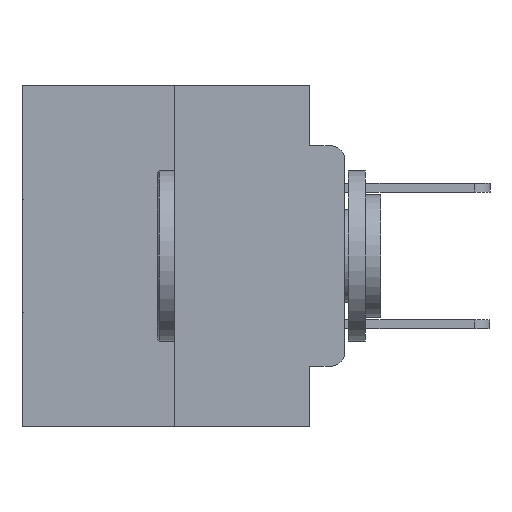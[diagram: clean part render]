
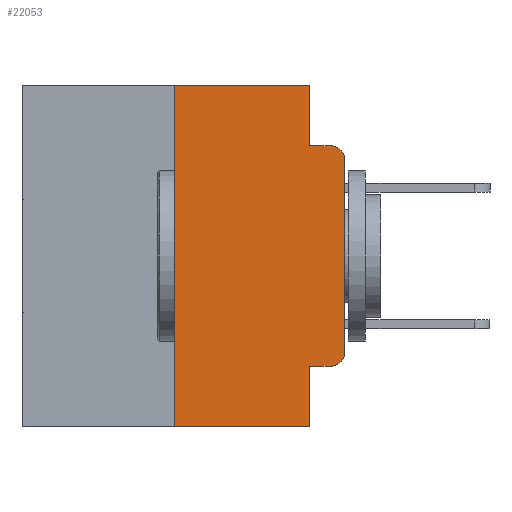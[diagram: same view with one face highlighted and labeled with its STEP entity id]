
A CAD part, left-side view. The second image highlights one B-rep face of the part: STEP entity #22053.
In plain terms, the highlighted planar face has unit normal (-1, 0, 0).
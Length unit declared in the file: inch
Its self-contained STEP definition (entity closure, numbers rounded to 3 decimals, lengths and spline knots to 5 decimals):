
#342 = EDGE_LOOP ( 'NONE', ( #15551, #16254, #22757, #11785, #12450, #8671, #27499, #22422, #17977, #758 ) ) ;
#758 = ORIENTED_EDGE ( 'NONE', *, *, #17374, .T. ) ;
#1546 = DIRECTION ( 'NONE',  ( -1., 0., 0. ) ) ;
#2364 = FACE_OUTER_BOUND ( 'NONE', #342, .T. ) ;
#2388 = EDGE_CURVE ( 'NONE', #22418, #22709, #19149, .T. ) ;
#2465 = VERTEX_POINT ( 'NONE', #24366 ) ;
#3047 = VERTEX_POINT ( 'NONE', #22172 ) ;
#3096 = EDGE_CURVE ( 'NONE', #23798, #15438, #18480, .T. ) ;
#3315 = CARTESIAN_POINT ( 'NONE',  ( 0., 0.051, 0. ) ) ;
#3863 = CARTESIAN_POINT ( 'NONE',  ( 0., 0.473, 0. ) ) ;
#3922 = EDGE_CURVE ( 'NONE', #22709, #2465, #4862, .T. ) ;
#4197 = CARTESIAN_POINT ( 'NONE',  ( 0., 0.051, -0.0885 ) ) ;
#4744 = AXIS2_PLACEMENT_3D ( 'NONE', #18377, #5075, #20560 ) ;
#4862 = CIRCLE ( 'NONE', #20282, 0.02 ) ;
#5075 = DIRECTION ( 'NONE',  ( -1., 0., 0. ) ) ;
#5249 = VECTOR ( 'NONE', #15201, 39.37008 ) ;
#6132 = VECTOR ( 'NONE', #8450, 39.37008 ) ;
#6475 = DIRECTION ( 'NONE',  ( 0., -1., 0. ) ) ;
#6972 = EDGE_CURVE ( 'NONE', #18510, #2465, #7589, .T. ) ;
#7490 = EDGE_CURVE ( 'NONE', #7613, #11094, #17935, .T. ) ;
#7589 = LINE ( 'NONE', #4197, #24434 ) ;
#7613 = VERTEX_POINT ( 'NONE', #28527 ) ;
#7895 = VECTOR ( 'NONE', #13419, 39.37008 ) ;
#8450 = DIRECTION ( 'NONE',  ( 0., -1., 0. ) ) ;
#8636 = CARTESIAN_POINT ( 'NONE',  ( 0., 0., 0. ) ) ;
#8671 = ORIENTED_EDGE ( 'NONE', *, *, #11474, .F. ) ;
#8853 = PLANE ( 'NONE',  #14910 ) ;
#8885 = VECTOR ( 'NONE', #16711, 39.37008 ) ;
#8913 = CARTESIAN_POINT ( 'NONE',  ( 0., 0., -0.1085 ) ) ;
#8957 = CARTESIAN_POINT ( 'NONE',  ( 0., 0.051, -0.5 ) ) ;
#9612 = DIRECTION ( 'NONE',  ( 0., 0., 1. ) ) ;
#10019 = EDGE_CURVE ( 'NONE', #11094, #18510, #19877, .T. ) ;
#11094 = VERTEX_POINT ( 'NONE', #26860 ) ;
#11159 = DIRECTION ( 'NONE',  ( 1., 0., 0. ) ) ;
#11474 = EDGE_CURVE ( 'NONE', #23798, #7613, #27956, .T. ) ;
#11785 = ORIENTED_EDGE ( 'NONE', *, *, #10019, .F. ) ;
#11928 = VECTOR ( 'NONE', #20236, 39.37008 ) ;
#12450 = ORIENTED_EDGE ( 'NONE', *, *, #7490, .F. ) ;
#12606 = VECTOR ( 'NONE', #9612, 39.37008 ) ;
#12943 = EDGE_CURVE ( 'NONE', #23839, #15438, #19624, .T. ) ;
#12982 = CARTESIAN_POINT ( 'NONE',  ( 0., 0.25, 0. ) ) ;
#13419 = DIRECTION ( 'NONE',  ( 0., 0., -1. ) ) ;
#14834 = CARTESIAN_POINT ( 'NONE',  ( 0., 0.051, -0.0885 ) ) ;
#14910 = AXIS2_PLACEMENT_3D ( 'NONE', #24271, #11159, #26454 ) ;
#15017 = CARTESIAN_POINT ( 'NONE',  ( 0., 0.02, -0.1085 ) ) ;
#15201 = DIRECTION ( 'NONE',  ( 0., 0., 1. ) ) ;
#15438 = VERTEX_POINT ( 'NONE', #8957 ) ;
#15551 = ORIENTED_EDGE ( 'NONE', *, *, #2388, .T. ) ;
#15555 = DIRECTION ( 'NONE',  ( 0., -1., 0. ) ) ;
#15620 = CARTESIAN_POINT ( 'NONE',  ( 0., 0.051, 0. ) ) ;
#15908 = EDGE_CURVE ( 'NONE', #23839, #3047, #22592, .T. ) ;
#16254 = ORIENTED_EDGE ( 'NONE', *, *, #3922, .T. ) ;
#16711 = DIRECTION ( 'NONE',  ( 0., 0., -1. ) ) ;
#17211 = DIRECTION ( 'NONE',  ( 0., 0., -1. ) ) ;
#17374 = EDGE_CURVE ( 'NONE', #3047, #22418, #19744, .T. ) ;
#17444 = VECTOR ( 'NONE', #15555, 39.37008 ) ;
#17935 = LINE ( 'NONE', #3863, #6132 ) ;
#17977 = ORIENTED_EDGE ( 'NONE', *, *, #15908, .T. ) ;
#18377 = CARTESIAN_POINT ( 'NONE',  ( 0., 0.02, -0.3915 ) ) ;
#18480 = LINE ( 'NONE', #23117, #11928 ) ;
#18510 = VERTEX_POINT ( 'NONE', #14834 ) ;
#19149 = LINE ( 'NONE', #8636, #12606 ) ;
#19624 = LINE ( 'NONE', #15620, #7895 ) ;
#19707 = CARTESIAN_POINT ( 'NONE',  ( 0., 0.051, -0.4115 ) ) ;
#19744 = CIRCLE ( 'NONE', #4744, 0.02 ) ;
#19877 = LINE ( 'NONE', #3315, #8885 ) ;
#20236 = DIRECTION ( 'NONE',  ( 0., -1., 0. ) ) ;
#20282 = AXIS2_PLACEMENT_3D ( 'NONE', #15017, #1546, #17211 ) ;
#20560 = DIRECTION ( 'NONE',  ( 0., 0., -1. ) ) ;
#22053 = ADVANCED_FACE ( 'NONE', ( #2364 ), #8853, .F. ) ;
#22172 = CARTESIAN_POINT ( 'NONE',  ( 0., 0.02, -0.4115 ) ) ;
#22418 = VERTEX_POINT ( 'NONE', #23130 ) ;
#22422 = ORIENTED_EDGE ( 'NONE', *, *, #12943, .F. ) ;
#22592 = LINE ( 'NONE', #24154, #17444 ) ;
#22709 = VERTEX_POINT ( 'NONE', #8913 ) ;
#22757 = ORIENTED_EDGE ( 'NONE', *, *, #6972, .F. ) ;
#23117 = CARTESIAN_POINT ( 'NONE',  ( 0., 0.473, -0.5 ) ) ;
#23130 = CARTESIAN_POINT ( 'NONE',  ( 0., 0., -0.3915 ) ) ;
#23798 = VERTEX_POINT ( 'NONE', #23993 ) ;
#23839 = VERTEX_POINT ( 'NONE', #19707 ) ;
#23993 = CARTESIAN_POINT ( 'NONE',  ( 0., 0.25, -0.5 ) ) ;
#24154 = CARTESIAN_POINT ( 'NONE',  ( 0., 0.051, -0.4115 ) ) ;
#24271 = CARTESIAN_POINT ( 'NONE',  ( 0., 0.473, 0. ) ) ;
#24366 = CARTESIAN_POINT ( 'NONE',  ( 0., 0.02, -0.0885 ) ) ;
#24434 = VECTOR ( 'NONE', #6475, 39.37008 ) ;
#26454 = DIRECTION ( 'NONE',  ( 0., 0., -1. ) ) ;
#26860 = CARTESIAN_POINT ( 'NONE',  ( 0., 0.051, 0. ) ) ;
#27499 = ORIENTED_EDGE ( 'NONE', *, *, #3096, .T. ) ;
#27956 = LINE ( 'NONE', #12982, #5249 ) ;
#28527 = CARTESIAN_POINT ( 'NONE',  ( 0., 0.25, 0. ) ) ;
